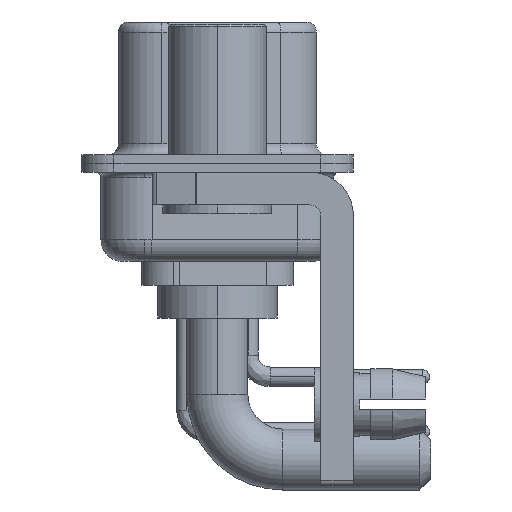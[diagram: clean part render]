
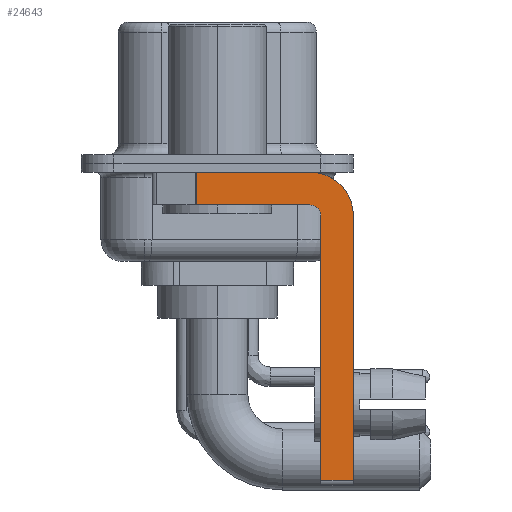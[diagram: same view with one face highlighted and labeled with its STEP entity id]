
A CAD part, left-side view. The second image highlights one B-rep face of the part: STEP entity #24643.
In plain terms, the highlighted planar face has unit normal (-1, 0, 0).
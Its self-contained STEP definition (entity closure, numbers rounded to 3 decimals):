
#280 = EDGE_CURVE ( 'NONE', #19555, #20987, #22991, .T. ) ;
#683 = VERTEX_POINT ( 'NONE', #1635 ) ;
#1432 = VECTOR ( 'NONE', #9961, 1000. ) ;
#1571 = CARTESIAN_POINT ( 'NONE',  ( -2.9, -4.25, -1.9 ) ) ;
#1635 = CARTESIAN_POINT ( 'NONE',  ( -2.9, 0.978, -0.4 ) ) ;
#1719 = AXIS2_PLACEMENT_3D ( 'NONE', #14571, #4017, #23880 ) ;
#1884 = LINE ( 'NONE', #4328, #7586 ) ;
#2258 = VERTEX_POINT ( 'NONE', #25808 ) ;
#2568 = CARTESIAN_POINT ( 'NONE',  ( -2.9, 0.978, -1.9 ) ) ;
#2625 = FACE_OUTER_BOUND ( 'NONE', #2892, .T. ) ;
#2645 = LINE ( 'NONE', #15920, #22885 ) ;
#2892 = EDGE_LOOP ( 'NONE', ( #10086, #6300, #16721, #7842, #11414, #27573, #7615, #21524 ) ) ;
#4017 = DIRECTION ( 'NONE',  ( -1., 0., 0. ) ) ;
#4328 = CARTESIAN_POINT ( 'NONE',  ( -2.9, -4.25, -14.55 ) ) ;
#4676 = VERTEX_POINT ( 'NONE', #14636 ) ;
#4901 = EDGE_CURVE ( 'NONE', #5462, #9564, #24929, .T. ) ;
#5234 = EDGE_CURVE ( 'NONE', #19555, #2258, #1884, .T. ) ;
#5462 = VERTEX_POINT ( 'NONE', #1571 ) ;
#6300 = ORIENTED_EDGE ( 'NONE', *, *, #18551, .T. ) ;
#7166 = VERTEX_POINT ( 'NONE', #26588 ) ;
#7212 = DIRECTION ( 'NONE',  ( 0., 0., -1. ) ) ;
#7586 = VECTOR ( 'NONE', #21774, 1000. ) ;
#7615 = ORIENTED_EDGE ( 'NONE', *, *, #13219, .F. ) ;
#7733 = CARTESIAN_POINT ( 'NONE',  ( -2.9, 3., -0.4 ) ) ;
#7842 = ORIENTED_EDGE ( 'NONE', *, *, #8063, .F. ) ;
#7882 = DIRECTION ( 'NONE',  ( 1., 0., 0. ) ) ;
#8063 = EDGE_CURVE ( 'NONE', #20987, #5462, #8103, .T. ) ;
#8103 = CIRCLE ( 'NONE', #1719, 0.5 ) ;
#8926 = DIRECTION ( 'NONE',  ( 0., 0., -1. ) ) ;
#9191 = CARTESIAN_POINT ( 'NONE',  ( -2.9, -4.25, -2.4 ) ) ;
#9564 = VERTEX_POINT ( 'NONE', #2568 ) ;
#9603 = CARTESIAN_POINT ( 'NONE',  ( -2.9, -4.25, -2.4 ) ) ;
#9759 = DIRECTION ( 'NONE',  ( 0., 1., 0. ) ) ;
#9961 = DIRECTION ( 'NONE',  ( 0., 0., 1. ) ) ;
#10025 = DIRECTION ( 'NONE',  ( 0., 0., -1. ) ) ;
#10086 = ORIENTED_EDGE ( 'NONE', *, *, #22944, .F. ) ;
#11331 = PLANE ( 'NONE',  #23308 ) ;
#11414 = ORIENTED_EDGE ( 'NONE', *, *, #280, .F. ) ;
#12191 = CIRCLE ( 'NONE', #28183, 2. ) ;
#13219 = EDGE_CURVE ( 'NONE', #4676, #2258, #24944, .T. ) ;
#13959 = VECTOR ( 'NONE', #9759, 1000. ) ;
#14165 = LINE ( 'NONE', #7733, #23291 ) ;
#14571 = CARTESIAN_POINT ( 'NONE',  ( -2.9, -4.25, -2.4 ) ) ;
#14636 = CARTESIAN_POINT ( 'NONE',  ( -2.9, -6.25, -2.4 ) ) ;
#15920 = CARTESIAN_POINT ( 'NONE',  ( -2.9, 0.978, -1.9 ) ) ;
#16721 = ORIENTED_EDGE ( 'NONE', *, *, #4901, .F. ) ;
#17901 = DIRECTION ( 'NONE',  ( 0., 0., -1. ) ) ;
#18551 = EDGE_CURVE ( 'NONE', #683, #9564, #2645, .T. ) ;
#19555 = VERTEX_POINT ( 'NONE', #22845 ) ;
#20312 = EDGE_CURVE ( 'NONE', #7166, #4676, #12191, .T. ) ;
#20613 = CARTESIAN_POINT ( 'NONE',  ( -2.9, -4.25, -1.9 ) ) ;
#20987 = VERTEX_POINT ( 'NONE', #22679 ) ;
#21524 = ORIENTED_EDGE ( 'NONE', *, *, #20312, .F. ) ;
#21774 = DIRECTION ( 'NONE',  ( 0., -1., 0. ) ) ;
#22523 = CARTESIAN_POINT ( 'NONE',  ( -2.9, -6.25, -2.4 ) ) ;
#22679 = CARTESIAN_POINT ( 'NONE',  ( -2.9, -4.75, -2.4 ) ) ;
#22845 = CARTESIAN_POINT ( 'NONE',  ( -2.9, -4.75, -14.55 ) ) ;
#22885 = VECTOR ( 'NONE', #8926, 1000. ) ;
#22921 = DIRECTION ( 'NONE',  ( 0., -1., 0. ) ) ;
#22944 = EDGE_CURVE ( 'NONE', #683, #7166, #14165, .T. ) ;
#22991 = LINE ( 'NONE', #23412, #1432 ) ;
#23291 = VECTOR ( 'NONE', #22921, 1000. ) ;
#23308 = AXIS2_PLACEMENT_3D ( 'NONE', #9191, #28225, #17901 ) ;
#23412 = CARTESIAN_POINT ( 'NONE',  ( -2.9, -4.75, -14.8 ) ) ;
#23880 = DIRECTION ( 'NONE',  ( 0., 0., 1. ) ) ;
#24643 = ADVANCED_FACE ( 'NONE', ( #2625 ), #11331, .F. ) ;
#24929 = LINE ( 'NONE', #20613, #13959 ) ;
#24944 = LINE ( 'NONE', #22523, #24972 ) ;
#24972 = VECTOR ( 'NONE', #7212, 1000. ) ;
#25808 = CARTESIAN_POINT ( 'NONE',  ( -2.9, -6.25, -14.55 ) ) ;
#26588 = CARTESIAN_POINT ( 'NONE',  ( -2.9, -4.25, -0.4 ) ) ;
#27573 = ORIENTED_EDGE ( 'NONE', *, *, #5234, .T. ) ;
#28183 = AXIS2_PLACEMENT_3D ( 'NONE', #9603, #7882, #10025 ) ;
#28225 = DIRECTION ( 'NONE',  ( 1., 0., 0. ) ) ;
